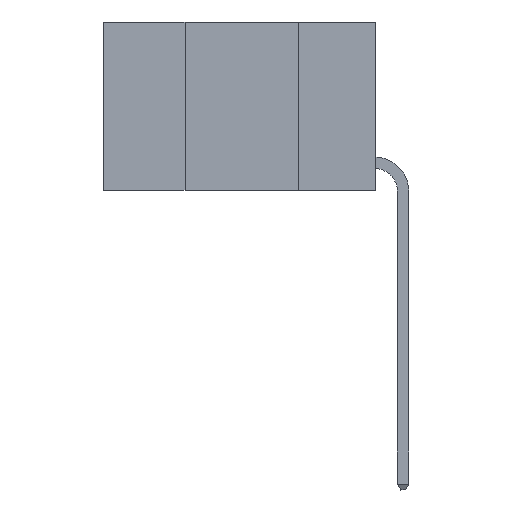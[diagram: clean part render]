
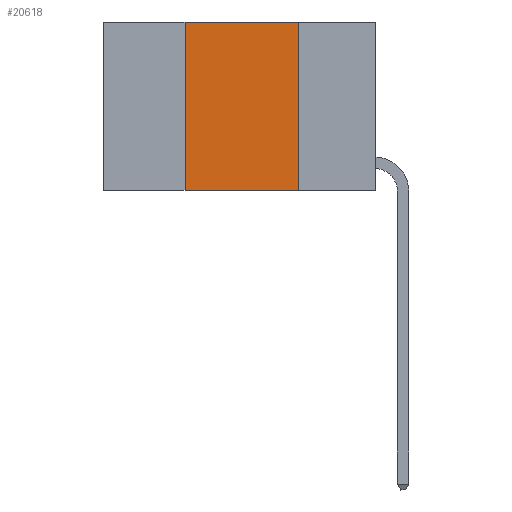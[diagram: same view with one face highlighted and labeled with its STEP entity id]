
A CAD part, left-side view. The second image highlights one B-rep face of the part: STEP entity #20618.
In plain terms, the highlighted planar face has unit normal (-1, 0, 0).
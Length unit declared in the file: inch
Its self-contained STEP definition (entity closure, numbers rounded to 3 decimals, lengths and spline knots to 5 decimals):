
#556 = PLANE ( 'NONE',  #19792 ) ;
#1643 = VERTEX_POINT ( 'NONE', #20932 ) ;
#2393 = CARTESIAN_POINT ( 'NONE',  ( 0., 0.6, 0. ) ) ;
#2949 = EDGE_CURVE ( 'NONE', #1643, #21310, #15569, .T. ) ;
#3889 = FACE_OUTER_BOUND ( 'NONE', #17061, .T. ) ;
#4131 = EDGE_CURVE ( 'NONE', #6672, #1643, #22421, .T. ) ;
#5615 = LINE ( 'NONE', #19598, #20854 ) ;
#6222 = EDGE_CURVE ( 'NONE', #21310, #9775, #22511, .T. ) ;
#6644 = CARTESIAN_POINT ( 'NONE',  ( 0., 0.17, 0. ) ) ;
#6672 = VERTEX_POINT ( 'NONE', #15722 ) ;
#7464 = DIRECTION ( 'NONE',  ( 0., -1., 0. ) ) ;
#8039 = CARTESIAN_POINT ( 'NONE',  ( 0., 0.17, -0.37 ) ) ;
#8578 = VECTOR ( 'NONE', #13695, 39.37008 ) ;
#8771 = DIRECTION ( 'NONE',  ( 0., -1., 0. ) ) ;
#9775 = VERTEX_POINT ( 'NONE', #8039 ) ;
#9782 = VECTOR ( 'NONE', #11507, 39.37008 ) ;
#10782 = DIRECTION ( 'NONE',  ( 0., 0., -1. ) ) ;
#11507 = DIRECTION ( 'NONE',  ( 0., 0., 1. ) ) ;
#13401 = ORIENTED_EDGE ( 'NONE', *, *, #18191, .T. ) ;
#13503 = ORIENTED_EDGE ( 'NONE', *, *, #4131, .F. ) ;
#13695 = DIRECTION ( 'NONE',  ( 0., 0., -1. ) ) ;
#14256 = DIRECTION ( 'NONE',  ( 1., 0., 0. ) ) ;
#14759 = ORIENTED_EDGE ( 'NONE', *, *, #6222, .F. ) ;
#15569 = LINE ( 'NONE', #17671, #19344 ) ;
#15722 = CARTESIAN_POINT ( 'NONE',  ( 0., 0.42, -0.37 ) ) ;
#16810 = ORIENTED_EDGE ( 'NONE', *, *, #2949, .F. ) ;
#17061 = EDGE_LOOP ( 'NONE', ( #14759, #16810, #13503, #13401 ) ) ;
#17671 = CARTESIAN_POINT ( 'NONE',  ( 0., 0.6, 0. ) ) ;
#18191 = EDGE_CURVE ( 'NONE', #6672, #9775, #5615, .T. ) ;
#18470 = CARTESIAN_POINT ( 'NONE',  ( 0., 0.42, 0. ) ) ;
#19163 = CARTESIAN_POINT ( 'NONE',  ( 0., 0.17, 0. ) ) ;
#19344 = VECTOR ( 'NONE', #8771, 39.37008 ) ;
#19598 = CARTESIAN_POINT ( 'NONE',  ( 0., 0.6, -0.37 ) ) ;
#19792 = AXIS2_PLACEMENT_3D ( 'NONE', #2393, #14256, #10782 ) ;
#20618 = ADVANCED_FACE ( 'NONE', ( #3889 ), #556, .F. ) ;
#20854 = VECTOR ( 'NONE', #7464, 39.37008 ) ;
#20932 = CARTESIAN_POINT ( 'NONE',  ( 0., 0.42, 0. ) ) ;
#21310 = VERTEX_POINT ( 'NONE', #19163 ) ;
#22421 = LINE ( 'NONE', #18470, #9782 ) ;
#22511 = LINE ( 'NONE', #6644, #8578 ) ;
